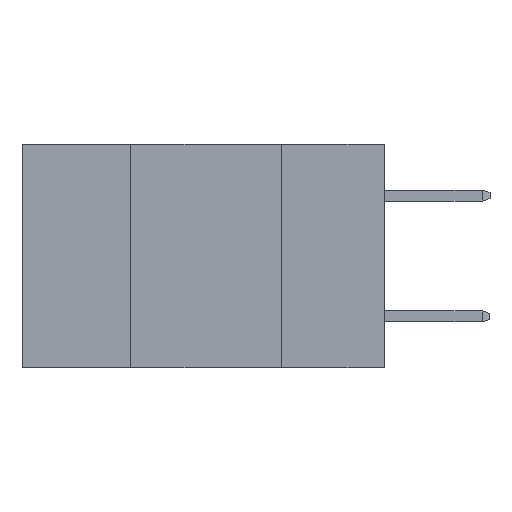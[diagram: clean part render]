
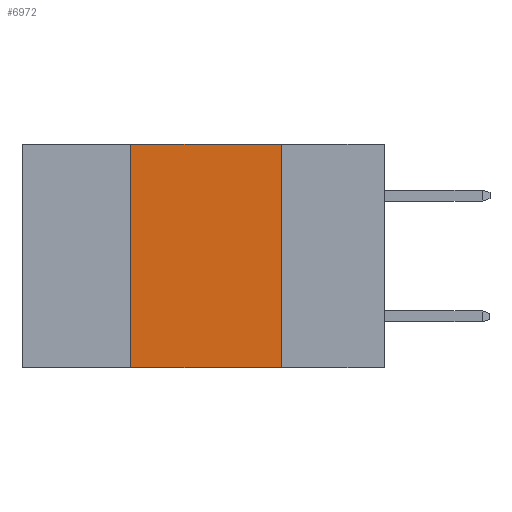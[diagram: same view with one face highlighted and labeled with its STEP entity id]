
A CAD part, left-side view. The second image highlights one B-rep face of the part: STEP entity #6972.
In plain terms, the highlighted planar face has unit normal (-1, 0, 0).
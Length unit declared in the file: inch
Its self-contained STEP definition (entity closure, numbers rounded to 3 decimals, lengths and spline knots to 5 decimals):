
#405 = CARTESIAN_POINT ( 'NONE',  ( 0., 0.6, 0. ) ) ;
#769 = DIRECTION ( 'NONE',  ( 0., 0., 1. ) ) ;
#1459 = ORIENTED_EDGE ( 'NONE', *, *, #2401, .T. ) ;
#1537 = LINE ( 'NONE', #4764, #4308 ) ;
#1616 = CARTESIAN_POINT ( 'NONE',  ( 0., 0.17, 0. ) ) ;
#1626 = EDGE_CURVE ( 'NONE', #6885, #3176, #4014, .T. ) ;
#1768 = ORIENTED_EDGE ( 'NONE', *, *, #9679, .F. ) ;
#1792 = DIRECTION ( 'NONE',  ( 0., 0., -1. ) ) ;
#1893 = LINE ( 'NONE', #2811, #4337 ) ;
#2401 = EDGE_CURVE ( 'NONE', #2791, #3176, #1537, .T. ) ;
#2574 = CARTESIAN_POINT ( 'NONE',  ( 0., 0.17, -0.37 ) ) ;
#2791 = VERTEX_POINT ( 'NONE', #3126 ) ;
#2811 = CARTESIAN_POINT ( 'NONE',  ( 0., 0.6, 0. ) ) ;
#2947 = CARTESIAN_POINT ( 'NONE',  ( 0., 0.42, 0. ) ) ;
#3126 = CARTESIAN_POINT ( 'NONE',  ( 0., 0.42, -0.37 ) ) ;
#3176 = VERTEX_POINT ( 'NONE', #2574 ) ;
#3200 = VECTOR ( 'NONE', #769, 39.37008 ) ;
#4014 = LINE ( 'NONE', #1616, #9251 ) ;
#4308 = VECTOR ( 'NONE', #8990, 39.37008 ) ;
#4337 = VECTOR ( 'NONE', #4917, 39.37008 ) ;
#4764 = CARTESIAN_POINT ( 'NONE',  ( 0., 0.6, -0.37 ) ) ;
#4917 = DIRECTION ( 'NONE',  ( 0., -1., 0. ) ) ;
#5641 = PLANE ( 'NONE',  #9189 ) ;
#5689 = DIRECTION ( 'NONE',  ( 1., 0., 0. ) ) ;
#6885 = VERTEX_POINT ( 'NONE', #7608 ) ;
#6972 = ADVANCED_FACE ( 'NONE', ( #7875 ), #5641, .F. ) ;
#7608 = CARTESIAN_POINT ( 'NONE',  ( 0., 0.17, 0. ) ) ;
#7875 = FACE_OUTER_BOUND ( 'NONE', #9651, .T. ) ;
#8990 = DIRECTION ( 'NONE',  ( 0., -1., 0. ) ) ;
#9158 = EDGE_CURVE ( 'NONE', #2791, #9793, #11446, .T. ) ;
#9189 = AXIS2_PLACEMENT_3D ( 'NONE', #405, #5689, #12786 ) ;
#9251 = VECTOR ( 'NONE', #1792, 39.37008 ) ;
#9380 = ORIENTED_EDGE ( 'NONE', *, *, #1626, .F. ) ;
#9651 = EDGE_LOOP ( 'NONE', ( #9380, #1768, #10870, #1459 ) ) ;
#9679 = EDGE_CURVE ( 'NONE', #9793, #6885, #1893, .T. ) ;
#9793 = VERTEX_POINT ( 'NONE', #2947 ) ;
#10870 = ORIENTED_EDGE ( 'NONE', *, *, #9158, .F. ) ;
#11446 = LINE ( 'NONE', #13070, #3200 ) ;
#12786 = DIRECTION ( 'NONE',  ( 0., 0., -1. ) ) ;
#13070 = CARTESIAN_POINT ( 'NONE',  ( 0., 0.42, 0. ) ) ;
